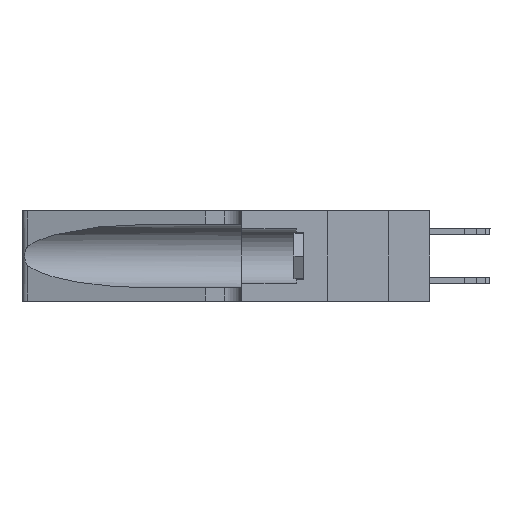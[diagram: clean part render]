
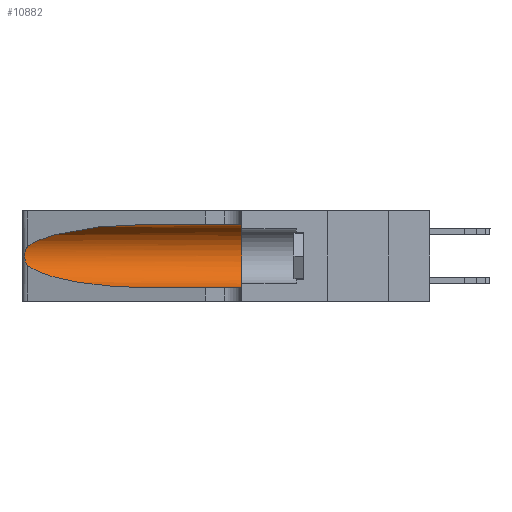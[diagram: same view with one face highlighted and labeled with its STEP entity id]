
A CAD part, left-side view. The second image highlights one B-rep face of the part: STEP entity #10882.
In plain terms, the highlighted cylindrical face has radius 3.308 mm (diameter 6.617 mm), a partial arc.
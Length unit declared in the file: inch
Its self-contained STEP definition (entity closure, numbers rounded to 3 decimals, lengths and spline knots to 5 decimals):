
#137 = CIRCLE ( 'NONE', #6226, 0.13025 ) ;
#143 = EDGE_CURVE ( 'NONE', #20388, #912, #12145, .T. ) ;
#238 = CARTESIAN_POINT ( 'NONE',  ( 0.1305, 0.35, 0.05475 ) ) ;
#912 = VERTEX_POINT ( 'NONE', #4151 ) ;
#1412 = DIRECTION ( 'NONE',  ( 0., -1., 0. ) ) ;
#1490 = CARTESIAN_POINT ( 'NONE',  ( 0.1305, 1.61858, 0.31525 ) ) ;
#3504 = CARTESIAN_POINT ( 'NONE',  ( 0.25487, 1.22718, 0.22369 ) ) ;
#3661 = EDGE_CURVE ( 'NONE', #8870, #15941, #14015, .T. ) ;
#3815 = CARTESIAN_POINT ( 'NONE',  ( 0.25555, 1.22993, 0.14849 ) ) ;
#4151 = CARTESIAN_POINT ( 'NONE',  ( 0.1305, 0.35, 0.31525 ) ) ;
#4238 = AXIS2_PLACEMENT_3D ( 'NONE', #10383, #8753, #18029 ) ;
#5397 = CARTESIAN_POINT ( 'NONE',  ( 0.1305, 0.72297, 0.05475 ) ) ;
#5459 = CARTESIAN_POINT ( 'NONE',  ( 0.25856, 1.23593, 0.16098 ) ) ;
#5543 = CARTESIAN_POINT ( 'NONE',  ( 0.25555, 1.22994, 0.2215 ) ) ;
#5973 = CARTESIAN_POINT ( 'NONE',  ( 0.1305, 0.35, 0.185 ) ) ;
#6226 = AXIS2_PLACEMENT_3D ( 'NONE', #5973, #22863, #6298 ) ;
#6298 = DIRECTION ( 'NONE',  ( 0., 0., 1. ) ) ;
#7140 = ORIENTED_EDGE ( 'NONE', *, *, #19984, .T. ) ;
#8464 = VERTEX_POINT ( 'NONE', #18931 ) ;
#8753 = DIRECTION ( 'NONE',  ( 0., -1., 0. ) ) ;
#8870 = VERTEX_POINT ( 'NONE', #5397 ) ;
#9024 =( BOUNDED_CURVE ( )  B_SPLINE_CURVE ( 3, ( #11030, #18292, #10949, #22206 ),
 .UNSPECIFIED., .F., .F. ) 
 B_SPLINE_CURVE_WITH_KNOTS ( ( 4, 4 ),
 ( 1.5708, 2.84003 ),
 .UNSPECIFIED. ) 
 CURVE ( )  GEOMETRIC_REPRESENTATION_ITEM ( )  RATIONAL_B_SPLINE_CURVE ( ( 1., 0.87, 0.87, 1. ) ) 
 REPRESENTATION_ITEM ( '' )  );
#9215 = CARTESIAN_POINT ( 'NONE',  ( 0.26075, 1.23896, 0.178 ) ) ;
#9347 = VERTEX_POINT ( 'NONE', #21421 ) ;
#10251 = VECTOR ( 'NONE', #23286, 39.37008 ) ;
#10383 = CARTESIAN_POINT ( 'NONE',  ( 0.1305, 1.61858, 0.185 ) ) ;
#10392 = EDGE_CURVE ( 'NONE', #20388, #9347, #9024, .T. ) ;
#10882 = ADVANCED_FACE ( 'NONE', ( #13675 ), #14267, .F. ) ;
#10903 = EDGE_LOOP ( 'NONE', ( #12961, #13936, #7140, #13089, #12009, #21280 ) ) ;
#10949 = CARTESIAN_POINT ( 'NONE',  ( 0.2373, 1.15595, 0.28018 ) ) ;
#11030 = CARTESIAN_POINT ( 'NONE',  ( 0.1305, 0.72297, 0.31525 ) ) ;
#11065 = CARTESIAN_POINT ( 'NONE',  ( 0.26075, 1.23896, 0.19203 ) ) ;
#11228 = CARTESIAN_POINT ( 'NONE',  ( 0.25787, 1.23484, 0.2124 ) ) ;
#11650 = EDGE_CURVE ( 'NONE', #9347, #8464, #20199, .T. ) ;
#12009 = ORIENTED_EDGE ( 'NONE', *, *, #19919, .F. ) ;
#12145 = LINE ( 'NONE', #1490, #16478 ) ;
#12961 = ORIENTED_EDGE ( 'NONE', *, *, #10392, .T. ) ;
#13089 = ORIENTED_EDGE ( 'NONE', *, *, #3661, .T. ) ;
#13675 = FACE_OUTER_BOUND ( 'NONE', #10903, .T. ) ;
#13691 = CARTESIAN_POINT ( 'NONE',  ( 0.1305, 0.72297, 0.31525 ) ) ;
#13869 = CARTESIAN_POINT ( 'NONE',  ( 0.25487, 1.22718, 0.14631 ) ) ;
#13936 = ORIENTED_EDGE ( 'NONE', *, *, #11650, .T. ) ;
#14015 = LINE ( 'NONE', #21308, #10251 ) ;
#14114 = CARTESIAN_POINT ( 'NONE',  ( 0.18966, 0.96281, 0.05475 ) ) ;
#14267 = CYLINDRICAL_SURFACE ( 'NONE', #4238, 0.13025 ) ;
#14654 = CARTESIAN_POINT ( 'NONE',  ( 0.25639, 1.23186, 0.15144 ) ) ;
#14819 = CARTESIAN_POINT ( 'NONE',  ( 0.25639, 1.23184, 0.21858 ) ) ;
#15562 =( BOUNDED_CURVE ( )  B_SPLINE_CURVE ( 3, ( #13869, #15740, #14114, #15895 ),
 .UNSPECIFIED., .F., .T. ) 
 B_SPLINE_CURVE_WITH_KNOTS ( ( 4, 4 ),
 ( 3.44316, 4.71239 ),
 .UNSPECIFIED. ) 
 CURVE ( )  GEOMETRIC_REPRESENTATION_ITEM ( )  RATIONAL_B_SPLINE_CURVE ( ( 1., 0.87, 0.87, 1. ) ) 
 REPRESENTATION_ITEM ( '' )  );
#15740 = CARTESIAN_POINT ( 'NONE',  ( 0.2373, 1.15595, 0.08982 ) ) ;
#15895 = CARTESIAN_POINT ( 'NONE',  ( 0.1305, 0.72297, 0.05475 ) ) ;
#15941 = VERTEX_POINT ( 'NONE', #238 ) ;
#16478 = VECTOR ( 'NONE', #1412, 39.37008 ) ;
#18029 = DIRECTION ( 'NONE',  ( 0., 0., -1. ) ) ;
#18292 = CARTESIAN_POINT ( 'NONE',  ( 0.18966, 0.96281, 0.31525 ) ) ;
#18397 = CARTESIAN_POINT ( 'NONE',  ( 0.26017, 1.23833, 0.17102 ) ) ;
#18713 = CARTESIAN_POINT ( 'NONE',  ( 0.26018, 1.23835, 0.19895 ) ) ;
#18931 = CARTESIAN_POINT ( 'NONE',  ( 0.25487, 1.22718, 0.14631 ) ) ;
#19919 = EDGE_CURVE ( 'NONE', #912, #15941, #137, .T. ) ;
#19984 = EDGE_CURVE ( 'NONE', #8464, #8870, #15562, .T. ) ;
#20199 = B_SPLINE_CURVE_WITH_KNOTS ( 'NONE', 3,
 ( #3504, #5543, #14819, #11228, #20594, #18713, #11065, #9215, #18397, #5459, #20511, #14654, #3815, #24132 ),
 .UNSPECIFIED., .F., .F.,
 ( 4, 2, 2, 2, 2, 2, 4 ),
 ( 0., 0.00027, 0.00053, 0.00107, 0.0016, 0.00187, 0.00214 ),
 .UNSPECIFIED. ) ;
#20388 = VERTEX_POINT ( 'NONE', #13691 ) ;
#20511 = CARTESIAN_POINT ( 'NONE',  ( 0.25789, 1.23486, 0.15765 ) ) ;
#20594 = CARTESIAN_POINT ( 'NONE',  ( 0.25854, 1.2359, 0.20912 ) ) ;
#21280 = ORIENTED_EDGE ( 'NONE', *, *, #143, .F. ) ;
#21308 = CARTESIAN_POINT ( 'NONE',  ( 0.1305, 1.61858, 0.05475 ) ) ;
#21421 = CARTESIAN_POINT ( 'NONE',  ( 0.25487, 1.22718, 0.22369 ) ) ;
#22206 = CARTESIAN_POINT ( 'NONE',  ( 0.25487, 1.22718, 0.22369 ) ) ;
#22863 = DIRECTION ( 'NONE',  ( 0., 1., 0. ) ) ;
#23286 = DIRECTION ( 'NONE',  ( 0., -1., 0. ) ) ;
#24132 = CARTESIAN_POINT ( 'NONE',  ( 0.25487, 1.22718, 0.14631 ) ) ;
